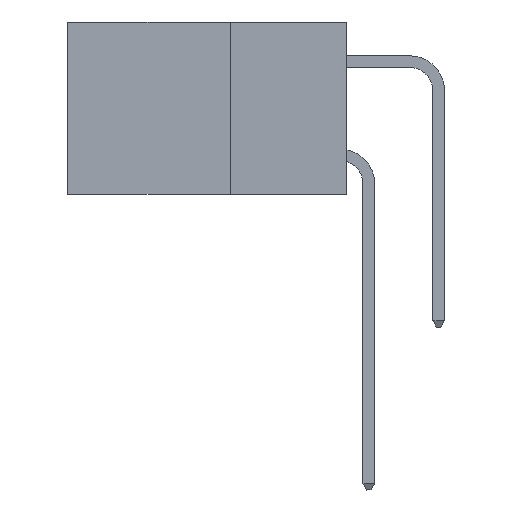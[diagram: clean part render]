
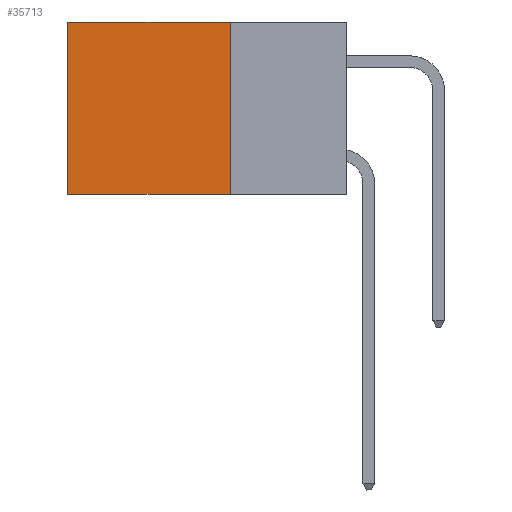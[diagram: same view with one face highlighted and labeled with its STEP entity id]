
A CAD part, left-side view. The second image highlights one B-rep face of the part: STEP entity #35713.
In plain terms, the highlighted planar face has unit normal (-1, 0, 0).
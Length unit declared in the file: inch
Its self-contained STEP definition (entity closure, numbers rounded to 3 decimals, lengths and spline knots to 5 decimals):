
#1483 = AXIS2_PLACEMENT_3D ( 'NONE', #27913, #7028, #13831 ) ;
#3340 = CARTESIAN_POINT ( 'NONE',  ( 0.2875, 0.6, 0. ) ) ;
#3566 = VECTOR ( 'NONE', #34872, 39.37008 ) ;
#3642 = DIRECTION ( 'NONE',  ( 0., 0., -1. ) ) ;
#6421 = VERTEX_POINT ( 'NONE', #14101 ) ;
#7028 = DIRECTION ( 'NONE',  ( 1., 0., 0. ) ) ;
#7374 = EDGE_CURVE ( 'NONE', #21182, #20016, #36893, .T. ) ;
#9686 = EDGE_CURVE ( 'NONE', #6421, #12249, #18278, .T. ) ;
#10145 = EDGE_CURVE ( 'NONE', #6421, #21182, #40948, .T. ) ;
#11493 = EDGE_CURVE ( 'NONE', #12249, #20016, #21973, .T. ) ;
#12249 = VERTEX_POINT ( 'NONE', #35058 ) ;
#13831 = DIRECTION ( 'NONE',  ( 0., 0., -1. ) ) ;
#14101 = CARTESIAN_POINT ( 'NONE',  ( 0.2875, 0.25, 0. ) ) ;
#18278 = LINE ( 'NONE', #26206, #43175 ) ;
#19519 = FACE_OUTER_BOUND ( 'NONE', #20109, .T. ) ;
#20016 = VERTEX_POINT ( 'NONE', #40302 ) ;
#20109 = EDGE_LOOP ( 'NONE', ( #24960, #39820, #29112, #30057 ) ) ;
#20988 = PLANE ( 'NONE',  #1483 ) ;
#21182 = VERTEX_POINT ( 'NONE', #21649 ) ;
#21649 = CARTESIAN_POINT ( 'NONE',  ( 0.2875, 0.6, 0. ) ) ;
#21973 = LINE ( 'NONE', #44262, #35987 ) ;
#24960 = ORIENTED_EDGE ( 'NONE', *, *, #7374, .T. ) ;
#26206 = CARTESIAN_POINT ( 'NONE',  ( 0.2875, 0.25, 0. ) ) ;
#26354 = DIRECTION ( 'NONE',  ( 0., 0., -1. ) ) ;
#26818 = DIRECTION ( 'NONE',  ( 0., 1., 0. ) ) ;
#27913 = CARTESIAN_POINT ( 'NONE',  ( 0.2875, 0.25, 0. ) ) ;
#29112 = ORIENTED_EDGE ( 'NONE', *, *, #9686, .F. ) ;
#30057 = ORIENTED_EDGE ( 'NONE', *, *, #10145, .T. ) ;
#31445 = VECTOR ( 'NONE', #3642, 39.37008 ) ;
#34872 = DIRECTION ( 'NONE',  ( 0., 1., 0. ) ) ;
#35058 = CARTESIAN_POINT ( 'NONE',  ( 0.2875, 0.25, -0.37 ) ) ;
#35713 = ADVANCED_FACE ( 'NONE', ( #19519 ), #20988, .F. ) ;
#35987 = VECTOR ( 'NONE', #26818, 39.37008 ) ;
#36893 = LINE ( 'NONE', #3340, #31445 ) ;
#38190 = CARTESIAN_POINT ( 'NONE',  ( 0.2875, 0.25, 0. ) ) ;
#39820 = ORIENTED_EDGE ( 'NONE', *, *, #11493, .F. ) ;
#40302 = CARTESIAN_POINT ( 'NONE',  ( 0.2875, 0.6, -0.37 ) ) ;
#40948 = LINE ( 'NONE', #38190, #3566 ) ;
#43175 = VECTOR ( 'NONE', #26354, 39.37008 ) ;
#44262 = CARTESIAN_POINT ( 'NONE',  ( 0.2875, 0.25, -0.37 ) ) ;
